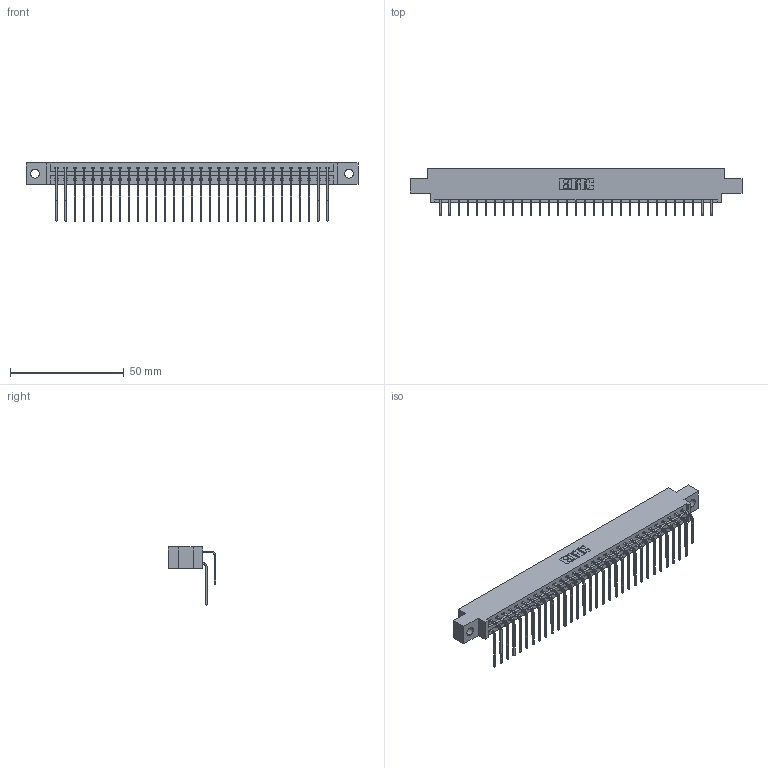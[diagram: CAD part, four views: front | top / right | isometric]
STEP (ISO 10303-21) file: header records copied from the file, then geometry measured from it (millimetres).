
FILE_DESCRIPTION (( 'STEP AP203' ), '1' );
FILE_NAME ('337-062-559-804.STEP', '2019-10-11T23:11:31', ( '' ), ( '' ), 'SwSTEP 2.0', 'SolidWorks 2016', '' );
FILE_SCHEMA (( 'CONFIG_CONTROL_DESIGN' ));
Length unit declared in the file: inch
Products named in the file (4): 345-292-001_558 559 Tail - 1; 345-292-001_559 Tail - 2; 337 Part_0.170 Offset - 0.156 Dia-TH; 337-062-559-804
Assembly tree (63 placements, depth 2):
  337-062-559-804
    337 Part_0.170 Offset - 0.156 Dia-TH
    345-292-001_558 559 Tail - 1  x31
    345-292-001_559 Tail - 2  x31
Bounding box: 145.85 x 20.9 x 25.53 mm (x, y, z)
Volume: 15376.4 mm3; surface area: 18977.3 mm2
Topology: 63 solids, 63 shells, 3590 faces, 10677 edges, 7034 vertices
Faces by surface type: plane 2554, cylinder 1036
Entity records: 27377 total; most frequent: CARTESIAN_POINT 4669, ORIENTED_EDGE 4554, DIRECTION 3973, EDGE_CURVE 2277, VECTOR 2109, LINE 2109, VERTEX_POINT 1514, AXIS2_PLACEMENT_3D 932
